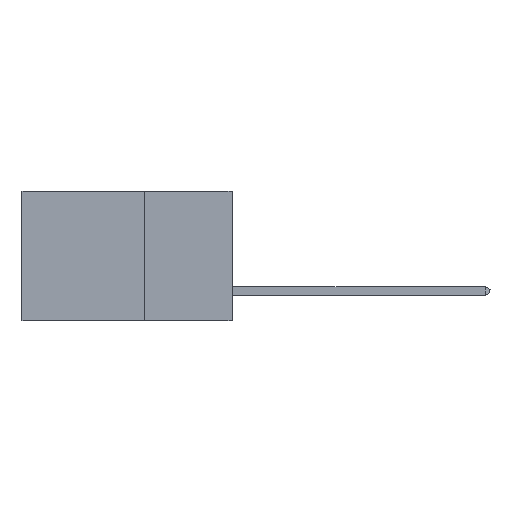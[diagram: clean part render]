
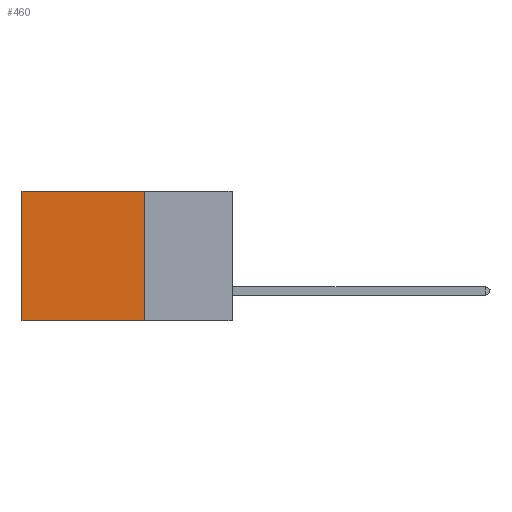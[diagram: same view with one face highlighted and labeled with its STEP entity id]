
A CAD part, left-side view. The second image highlights one B-rep face of the part: STEP entity #460.
In plain terms, the highlighted planar face has unit normal (-1, 0, 0).
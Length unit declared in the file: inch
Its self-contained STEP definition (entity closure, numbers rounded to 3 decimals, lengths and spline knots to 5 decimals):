
#336 = ORIENTED_EDGE ( 'NONE', *, *, #33537, .T. ) ;
#460 = ADVANCED_FACE ( 'NONE', ( #32447 ), #30966, .F. ) ;
#615 = EDGE_CURVE ( 'NONE', #39090, #39924, #4355, .T. ) ;
#1973 = VECTOR ( 'NONE', #30337, 39.37008 ) ;
#2872 = CARTESIAN_POINT ( 'NONE',  ( 0.2875, 0.25, -0.37 ) ) ;
#3603 = CARTESIAN_POINT ( 'NONE',  ( 0.2875, 0.25, 0. ) ) ;
#4355 = LINE ( 'NONE', #3603, #1973 ) ;
#4387 = DIRECTION ( 'NONE',  ( 0., 0., -1. ) ) ;
#5509 = CARTESIAN_POINT ( 'NONE',  ( 0.2875, 0.6, 0. ) ) ;
#6070 = DIRECTION ( 'NONE',  ( 0., 0., -1. ) ) ;
#7066 = LINE ( 'NONE', #43556, #35561 ) ;
#10871 = EDGE_CURVE ( 'NONE', #39924, #17132, #28709, .T. ) ;
#11528 = AXIS2_PLACEMENT_3D ( 'NONE', #16065, #46217, #4387 ) ;
#11967 = VECTOR ( 'NONE', #41193, 39.37008 ) ;
#11990 = CARTESIAN_POINT ( 'NONE',  ( 0.2875, 0.25, 0. ) ) ;
#15283 = ORIENTED_EDGE ( 'NONE', *, *, #26883, .T. ) ;
#16065 = CARTESIAN_POINT ( 'NONE',  ( 0.2875, 0.25, 0. ) ) ;
#17132 = VERTEX_POINT ( 'NONE', #32998 ) ;
#19434 = EDGE_LOOP ( 'NONE', ( #15283, #20581, #28554, #336 ) ) ;
#20581 = ORIENTED_EDGE ( 'NONE', *, *, #10871, .F. ) ;
#23591 = CARTESIAN_POINT ( 'NONE',  ( 0.2875, 0.25, -0.37 ) ) ;
#26883 = EDGE_CURVE ( 'NONE', #27258, #17132, #48609, .T. ) ;
#27258 = VERTEX_POINT ( 'NONE', #29181 ) ;
#28554 = ORIENTED_EDGE ( 'NONE', *, *, #615, .F. ) ;
#28709 = LINE ( 'NONE', #2872, #11967 ) ;
#29181 = CARTESIAN_POINT ( 'NONE',  ( 0.2875, 0.6, 0. ) ) ;
#30337 = DIRECTION ( 'NONE',  ( 0., 0., -1. ) ) ;
#30966 = PLANE ( 'NONE',  #11528 ) ;
#32447 = FACE_OUTER_BOUND ( 'NONE', #19434, .T. ) ;
#32998 = CARTESIAN_POINT ( 'NONE',  ( 0.2875, 0.6, -0.37 ) ) ;
#33537 = EDGE_CURVE ( 'NONE', #39090, #27258, #7066, .T. ) ;
#35561 = VECTOR ( 'NONE', #45970, 39.37008 ) ;
#39090 = VERTEX_POINT ( 'NONE', #11990 ) ;
#39924 = VERTEX_POINT ( 'NONE', #23591 ) ;
#41193 = DIRECTION ( 'NONE',  ( 0., 1., 0. ) ) ;
#43556 = CARTESIAN_POINT ( 'NONE',  ( 0.2875, 0.25, 0. ) ) ;
#45970 = DIRECTION ( 'NONE',  ( 0., 1., 0. ) ) ;
#46217 = DIRECTION ( 'NONE',  ( 1., 0., 0. ) ) ;
#47976 = VECTOR ( 'NONE', #6070, 39.37008 ) ;
#48609 = LINE ( 'NONE', #5509, #47976 ) ;
